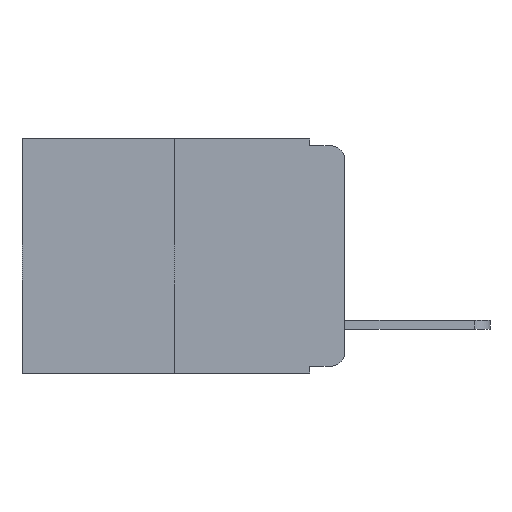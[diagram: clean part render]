
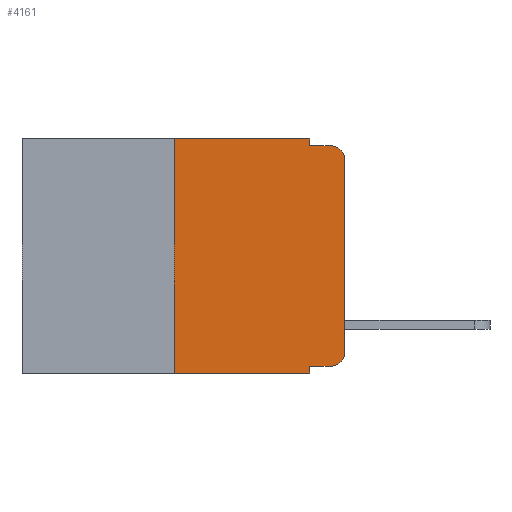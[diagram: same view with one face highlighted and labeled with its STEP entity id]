
A CAD part, left-side view. The second image highlights one B-rep face of the part: STEP entity #4161.
In plain terms, the highlighted planar face has unit normal (-1, 0, 0).
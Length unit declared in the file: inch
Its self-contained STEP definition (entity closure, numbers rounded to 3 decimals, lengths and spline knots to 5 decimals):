
#128 = DIRECTION ( 'NONE',  ( 0., 0., -1. ) ) ;
#142 = CARTESIAN_POINT ( 'NONE',  ( 0., 0.051, 0. ) ) ;
#401 = LINE ( 'NONE', #142, #10873 ) ;
#432 = VERTEX_POINT ( 'NONE', #9138 ) ;
#643 = DIRECTION ( 'NONE',  ( -1., 0., 0. ) ) ;
#754 = VECTOR ( 'NONE', #4908, 39.37008 ) ;
#930 = VERTEX_POINT ( 'NONE', #4845 ) ;
#970 = CARTESIAN_POINT ( 'NONE',  ( 0., 0.473, 0. ) ) ;
#1176 = CARTESIAN_POINT ( 'NONE',  ( 0., 0.051, -0.343 ) ) ;
#1208 = CARTESIAN_POINT ( 'NONE',  ( 0., 0.473, -0.343 ) ) ;
#1551 = CARTESIAN_POINT ( 'NONE',  ( 0., 0., 0. ) ) ;
#1581 = CIRCLE ( 'NONE', #1890, 0.02 ) ;
#1786 = DIRECTION ( 'NONE',  ( 0., 0., -1. ) ) ;
#1806 = CARTESIAN_POINT ( 'NONE',  ( 0., 0.051, 0. ) ) ;
#1838 = CARTESIAN_POINT ( 'NONE',  ( 0., 0.25, 0. ) ) ;
#1890 = AXIS2_PLACEMENT_3D ( 'NONE', #6536, #643, #7524 ) ;
#2137 = VERTEX_POINT ( 'NONE', #3068 ) ;
#2261 = DIRECTION ( 'NONE',  ( 0., -1., 0. ) ) ;
#2328 = CARTESIAN_POINT ( 'NONE',  ( 0., 0.051, -0.01 ) ) ;
#2392 = VECTOR ( 'NONE', #1786, 39.37008 ) ;
#2712 = LINE ( 'NONE', #1806, #2392 ) ;
#2790 = VERTEX_POINT ( 'NONE', #3525 ) ;
#3029 = EDGE_CURVE ( 'NONE', #2790, #4275, #2712, .T. ) ;
#3068 = CARTESIAN_POINT ( 'NONE',  ( 0., 0.25, -0.343 ) ) ;
#3387 = VECTOR ( 'NONE', #2261, 39.37008 ) ;
#3525 = CARTESIAN_POINT ( 'NONE',  ( 0., 0.051, 0. ) ) ;
#3721 = ORIENTED_EDGE ( 'NONE', *, *, #10552, .T. ) ;
#3878 = EDGE_CURVE ( 'NONE', #2137, #8359, #8525, .T. ) ;
#4104 = EDGE_CURVE ( 'NONE', #2137, #12543, #5393, .T. ) ;
#4161 = ADVANCED_FACE ( 'NONE', ( #11852 ), #12497, .F. ) ;
#4186 = ORIENTED_EDGE ( 'NONE', *, *, #10146, .T. ) ;
#4275 = VERTEX_POINT ( 'NONE', #7787 ) ;
#4472 = ORIENTED_EDGE ( 'NONE', *, *, #9481, .F. ) ;
#4845 = CARTESIAN_POINT ( 'NONE',  ( 0., 0.051, -0.333 ) ) ;
#4908 = DIRECTION ( 'NONE',  ( 0., -1., 0. ) ) ;
#4941 = CARTESIAN_POINT ( 'NONE',  ( 0., 0.051, -0.333 ) ) ;
#5157 = ORIENTED_EDGE ( 'NONE', *, *, #3029, .F. ) ;
#5318 = ORIENTED_EDGE ( 'NONE', *, *, #7128, .F. ) ;
#5336 = CARTESIAN_POINT ( 'NONE',  ( 0., 0.02, -0.333 ) ) ;
#5393 = LINE ( 'NONE', #1838, #12141 ) ;
#5778 = AXIS2_PLACEMENT_3D ( 'NONE', #970, #11653, #9893 ) ;
#5967 = VECTOR ( 'NONE', #9614, 39.37008 ) ;
#6201 = EDGE_LOOP ( 'NONE', ( #3721, #4186, #4472, #5157, #5318, #6642, #6768, #7827, #8154, #9738 ) ) ;
#6369 = DIRECTION ( 'NONE',  ( 0., 0., 1. ) ) ;
#6489 = LINE ( 'NONE', #11578, #11368 ) ;
#6536 = CARTESIAN_POINT ( 'NONE',  ( 0., 0.02, -0.03 ) ) ;
#6642 = ORIENTED_EDGE ( 'NONE', *, *, #4104, .F. ) ;
#6768 = ORIENTED_EDGE ( 'NONE', *, *, #3878, .T. ) ;
#7128 = EDGE_CURVE ( 'NONE', #12543, #2790, #6489, .T. ) ;
#7313 = LINE ( 'NONE', #1551, #12420 ) ;
#7459 = CARTESIAN_POINT ( 'NONE',  ( 0., 0., -0.03 ) ) ;
#7524 = DIRECTION ( 'NONE',  ( 0., 0., -1. ) ) ;
#7787 = CARTESIAN_POINT ( 'NONE',  ( 0., 0.051, -0.01 ) ) ;
#7826 = VERTEX_POINT ( 'NONE', #5336 ) ;
#7827 = ORIENTED_EDGE ( 'NONE', *, *, #9701, .F. ) ;
#7833 = CIRCLE ( 'NONE', #11313, 0.02 ) ;
#8118 = LINE ( 'NONE', #2328, #3387 ) ;
#8154 = ORIENTED_EDGE ( 'NONE', *, *, #9266, .T. ) ;
#8229 = VERTEX_POINT ( 'NONE', #7459 ) ;
#8359 = VERTEX_POINT ( 'NONE', #1176 ) ;
#8376 = EDGE_CURVE ( 'NONE', #7826, #432, #7833, .T. ) ;
#8525 = LINE ( 'NONE', #1208, #5967 ) ;
#8570 = LINE ( 'NONE', #4941, #754 ) ;
#9138 = CARTESIAN_POINT ( 'NONE',  ( 0., 0., -0.313 ) ) ;
#9266 = EDGE_CURVE ( 'NONE', #930, #7826, #8570, .T. ) ;
#9481 = EDGE_CURVE ( 'NONE', #4275, #11706, #8118, .T. ) ;
#9511 = CARTESIAN_POINT ( 'NONE',  ( 0., 0.25, 0. ) ) ;
#9614 = DIRECTION ( 'NONE',  ( 0., -1., 0. ) ) ;
#9701 = EDGE_CURVE ( 'NONE', #930, #8359, #401, .T. ) ;
#9738 = ORIENTED_EDGE ( 'NONE', *, *, #8376, .T. ) ;
#9893 = DIRECTION ( 'NONE',  ( 0., 0., -1. ) ) ;
#10146 = EDGE_CURVE ( 'NONE', #8229, #11706, #1581, .T. ) ;
#10319 = CARTESIAN_POINT ( 'NONE',  ( 0., 0.02, -0.01 ) ) ;
#10552 = EDGE_CURVE ( 'NONE', #432, #8229, #7313, .T. ) ;
#10873 = VECTOR ( 'NONE', #128, 39.37008 ) ;
#11313 = AXIS2_PLACEMENT_3D ( 'NONE', #12541, #11379, #12533 ) ;
#11368 = VECTOR ( 'NONE', #11527, 39.37008 ) ;
#11379 = DIRECTION ( 'NONE',  ( -1., 0., 0. ) ) ;
#11527 = DIRECTION ( 'NONE',  ( 0., -1., 0. ) ) ;
#11578 = CARTESIAN_POINT ( 'NONE',  ( 0., 0.473, 0. ) ) ;
#11653 = DIRECTION ( 'NONE',  ( 1., 0., 0. ) ) ;
#11706 = VERTEX_POINT ( 'NONE', #10319 ) ;
#11852 = FACE_OUTER_BOUND ( 'NONE', #6201, .T. ) ;
#12141 = VECTOR ( 'NONE', #12172, 39.37008 ) ;
#12172 = DIRECTION ( 'NONE',  ( 0., 0., 1. ) ) ;
#12420 = VECTOR ( 'NONE', #6369, 39.37008 ) ;
#12497 = PLANE ( 'NONE',  #5778 ) ;
#12533 = DIRECTION ( 'NONE',  ( 0., 0., -1. ) ) ;
#12541 = CARTESIAN_POINT ( 'NONE',  ( 0., 0.02, -0.313 ) ) ;
#12543 = VERTEX_POINT ( 'NONE', #9511 ) ;
